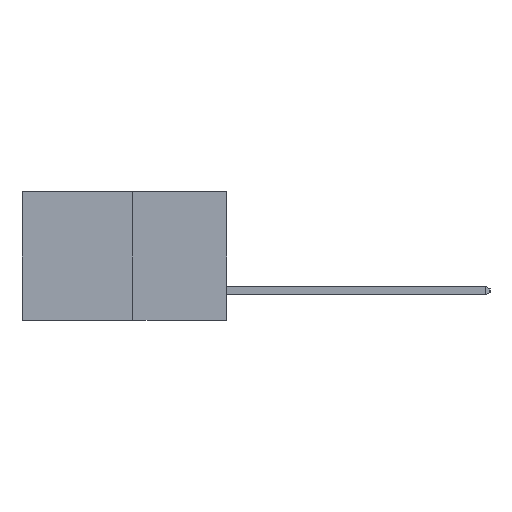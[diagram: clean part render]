
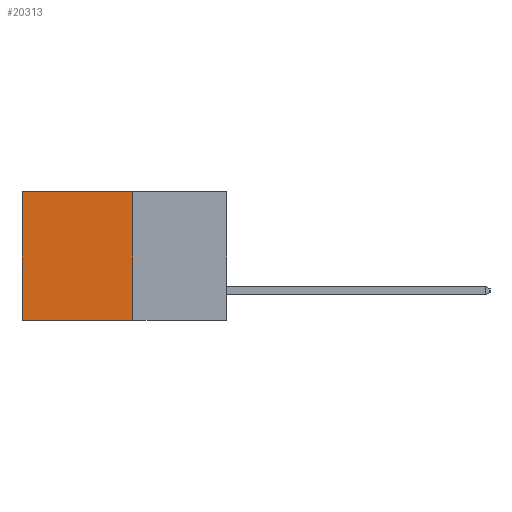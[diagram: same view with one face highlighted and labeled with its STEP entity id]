
A CAD part, left-side view. The second image highlights one B-rep face of the part: STEP entity #20313.
In plain terms, the highlighted planar face has unit normal (-1, 0, 0).
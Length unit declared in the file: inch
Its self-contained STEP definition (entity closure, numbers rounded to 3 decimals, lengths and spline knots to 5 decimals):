
#997 = CARTESIAN_POINT ( 'NONE',  ( 0.277, 0.27, -0.37 ) ) ;
#1751 = VECTOR ( 'NONE', #10174, 39.37008 ) ;
#2204 = VECTOR ( 'NONE', #3278, 39.37008 ) ;
#2406 = EDGE_CURVE ( 'NONE', #8947, #15704, #6531, .T. ) ;
#3278 = DIRECTION ( 'NONE',  ( 0., 0., -1. ) ) ;
#3802 = CARTESIAN_POINT ( 'NONE',  ( 0.277, 0.59, -0.37 ) ) ;
#4482 = ORIENTED_EDGE ( 'NONE', *, *, #15525, .T. ) ;
#6531 = LINE ( 'NONE', #14315, #2204 ) ;
#6670 = ORIENTED_EDGE ( 'NONE', *, *, #2406, .T. ) ;
#7705 = CARTESIAN_POINT ( 'NONE',  ( 0.277, 0.27, -0.37 ) ) ;
#8906 = EDGE_CURVE ( 'NONE', #12268, #12420, #11561, .T. ) ;
#8947 = VERTEX_POINT ( 'NONE', #12193 ) ;
#9119 = CARTESIAN_POINT ( 'NONE',  ( 0.277, 0.27, 0. ) ) ;
#9565 = DIRECTION ( 'NONE',  ( 0., 0., -1. ) ) ;
#10174 = DIRECTION ( 'NONE',  ( 0., 0., -1. ) ) ;
#10722 = ORIENTED_EDGE ( 'NONE', *, *, #21335, .F. ) ;
#11561 = LINE ( 'NONE', #997, #1751 ) ;
#12193 = CARTESIAN_POINT ( 'NONE',  ( 0.277, 0.59, 0. ) ) ;
#12268 = VERTEX_POINT ( 'NONE', #9119 ) ;
#12420 = VERTEX_POINT ( 'NONE', #15102 ) ;
#13116 = LINE ( 'NONE', #22951, #22686 ) ;
#13758 = DIRECTION ( 'NONE',  ( 0., 1., 0. ) ) ;
#14315 = CARTESIAN_POINT ( 'NONE',  ( 0.277, 0.59, -0.37 ) ) ;
#14706 = VECTOR ( 'NONE', #16163, 39.37008 ) ;
#15102 = CARTESIAN_POINT ( 'NONE',  ( 0.277, 0.27, -0.37 ) ) ;
#15292 = AXIS2_PLACEMENT_3D ( 'NONE', #7705, #20628, #9565 ) ;
#15525 = EDGE_CURVE ( 'NONE', #12268, #8947, #13116, .T. ) ;
#15704 = VERTEX_POINT ( 'NONE', #3802 ) ;
#16163 = DIRECTION ( 'NONE',  ( 0., 1., 0. ) ) ;
#17643 = EDGE_LOOP ( 'NONE', ( #6670, #10722, #23028, #4482 ) ) ;
#18240 = FACE_OUTER_BOUND ( 'NONE', #17643, .T. ) ;
#18798 = PLANE ( 'NONE',  #15292 ) ;
#19627 = LINE ( 'NONE', #23418, #14706 ) ;
#20313 = ADVANCED_FACE ( 'NONE', ( #18240 ), #18798, .F. ) ;
#20628 = DIRECTION ( 'NONE',  ( 1., 0., 0. ) ) ;
#21335 = EDGE_CURVE ( 'NONE', #12420, #15704, #19627, .T. ) ;
#22686 = VECTOR ( 'NONE', #13758, 39.37008 ) ;
#22951 = CARTESIAN_POINT ( 'NONE',  ( 0.277, 0.27, 0. ) ) ;
#23028 = ORIENTED_EDGE ( 'NONE', *, *, #8906, .F. ) ;
#23418 = CARTESIAN_POINT ( 'NONE',  ( 0.277, 0.27, -0.37 ) ) ;
